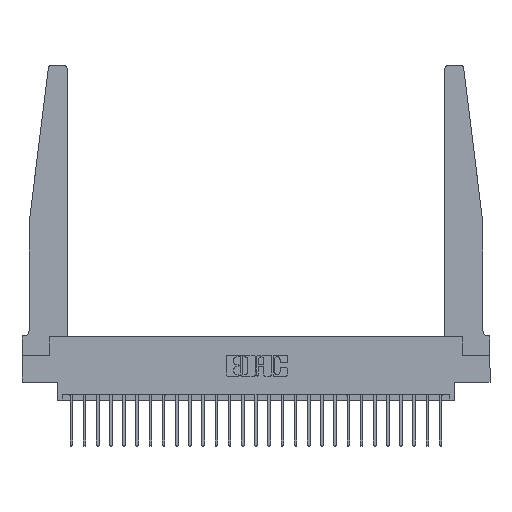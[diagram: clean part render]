
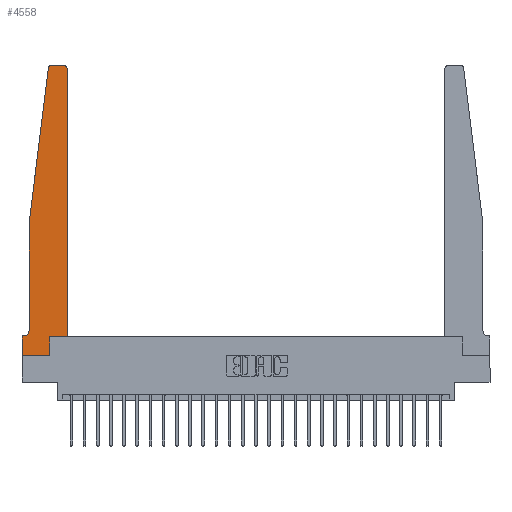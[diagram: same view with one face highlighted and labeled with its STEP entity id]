
A CAD part, top view. The second image highlights one B-rep face of the part: STEP entity #4558.
In plain terms, the highlighted planar face has unit normal (0, 0, 1).
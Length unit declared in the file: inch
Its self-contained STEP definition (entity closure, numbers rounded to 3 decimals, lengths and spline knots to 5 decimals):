
#84 = LINE ( 'NONE', #6139, #25958 ) ;
#349 = DIRECTION ( 'NONE',  ( 0., 0., -1. ) ) ;
#415 = CARTESIAN_POINT ( 'NONE',  ( 0.2605, 0.18, 0.37 ) ) ;
#795 = DIRECTION ( 'NONE',  ( 1., 0., 0. ) ) ;
#845 = VERTEX_POINT ( 'NONE', #19934 ) ;
#1404 = DIRECTION ( 'NONE',  ( 0., 0., 1. ) ) ;
#1995 = CIRCLE ( 'NONE', #16306, 0.03 ) ;
#2336 = CARTESIAN_POINT ( 'NONE',  ( 0.2605, 0.18, 0.37 ) ) ;
#2342 = CARTESIAN_POINT ( 'NONE',  ( 0.27653, 2.75, 0.37 ) ) ;
#2404 = ORIENTED_EDGE ( 'NONE', *, *, #10824, .T. ) ;
#3598 = VECTOR ( 'NONE', #15626, 39.37008 ) ;
#3661 = EDGE_CURVE ( 'NONE', #4424, #20110, #20264, .T. ) ;
#3955 = ORIENTED_EDGE ( 'NONE', *, *, #22838, .T. ) ;
#4188 = DIRECTION ( 'NONE',  ( 0., 1., 0. ) ) ;
#4293 = VECTOR ( 'NONE', #20482, 39.37008 ) ;
#4340 = EDGE_CURVE ( 'NONE', #5975, #11841, #15081, .T. ) ;
#4424 = VERTEX_POINT ( 'NONE', #20037 ) ;
#4433 = CARTESIAN_POINT ( 'NONE',  ( 0.395, 2.75, 0.37 ) ) ;
#4449 = CARTESIAN_POINT ( 'NONE',  ( 0.015, 0.1875, 0.37 ) ) ;
#4558 = ADVANCED_FACE ( 'NONE', ( #22544 ), #24651, .T. ) ;
#4831 = LINE ( 'NONE', #10779, #14802 ) ;
#5114 = VERTEX_POINT ( 'NONE', #4449 ) ;
#5836 = CARTESIAN_POINT ( 'NONE',  ( 0.065, 0.1875, 0.37 ) ) ;
#5975 = VERTEX_POINT ( 'NONE', #4433 ) ;
#6001 = DIRECTION ( 'NONE',  ( 0., -1., 0. ) ) ;
#6057 = CARTESIAN_POINT ( 'NONE',  ( 0.425, 2.72, 0.37 ) ) ;
#6135 = EDGE_CURVE ( 'NONE', #23276, #5975, #12417, .T. ) ;
#6139 = CARTESIAN_POINT ( 'NONE',  ( 0., 0., 0.37 ) ) ;
#6272 = DIRECTION ( 'NONE',  ( -1., 0., 0. ) ) ;
#6506 = CARTESIAN_POINT ( 'NONE',  ( 0.065, 1.25, 0.37 ) ) ;
#6802 = VERTEX_POINT ( 'NONE', #7889 ) ;
#6846 = DIRECTION ( 'NONE',  ( 0., 0., 1. ) ) ;
#7079 = DIRECTION ( 'NONE',  ( 0., 1., 0. ) ) ;
#7572 = DIRECTION ( 'NONE',  ( 1., 0., 0. ) ) ;
#7683 = LINE ( 'NONE', #15757, #3598 ) ;
#7856 = VERTEX_POINT ( 'NONE', #21136 ) ;
#7889 = CARTESIAN_POINT ( 'NONE',  ( 0.065, 1.25, 0.37 ) ) ;
#7890 = VECTOR ( 'NONE', #14556, 39.37008 ) ;
#9022 = VERTEX_POINT ( 'NONE', #21777 ) ;
#9404 = DIRECTION ( 'NONE',  ( -1., 0., 0. ) ) ;
#9525 = CIRCLE ( 'NONE', #19628, 0.05 ) ;
#9925 = ORIENTED_EDGE ( 'NONE', *, *, #20898, .T. ) ;
#10779 = CARTESIAN_POINT ( 'NONE',  ( 0.425, 0.18, 0.37 ) ) ;
#10824 = EDGE_CURVE ( 'NONE', #24375, #23276, #4831, .T. ) ;
#11055 = ORIENTED_EDGE ( 'NONE', *, *, #20810, .T. ) ;
#11338 = EDGE_CURVE ( 'NONE', #22339, #6802, #18080, .T. ) ;
#11629 = ORIENTED_EDGE ( 'NONE', *, *, #6135, .T. ) ;
#11781 = LINE ( 'NONE', #5836, #16328 ) ;
#11841 = VERTEX_POINT ( 'NONE', #2342 ) ;
#12039 = LINE ( 'NONE', #16641, #7890 ) ;
#12293 = VECTOR ( 'NONE', #4188, 39.37008 ) ;
#12417 = CIRCLE ( 'NONE', #15789, 0.03 ) ;
#13108 = ORIENTED_EDGE ( 'NONE', *, *, #22732, .T. ) ;
#13673 = EDGE_CURVE ( 'NONE', #6802, #7856, #14440, .T. ) ;
#13743 = CARTESIAN_POINT ( 'NONE',  ( 0.065, 1.25, 0.37 ) ) ;
#13976 = VECTOR ( 'NONE', #19778, 39.37008 ) ;
#14281 = ORIENTED_EDGE ( 'NONE', *, *, #11338, .T. ) ;
#14440 = LINE ( 'NONE', #6506, #4293 ) ;
#14556 = DIRECTION ( 'NONE',  ( 1., 0., 0. ) ) ;
#14802 = VECTOR ( 'NONE', #7079, 39.37008 ) ;
#15081 = LINE ( 'NONE', #25474, #25430 ) ;
#15377 = CARTESIAN_POINT ( 'NONE',  ( 0.395, 2.72, 0.37 ) ) ;
#15550 = CARTESIAN_POINT ( 'NONE',  ( 0.27653, 2.72, 0.37 ) ) ;
#15626 = DIRECTION ( 'NONE',  ( 1., 0., 0. ) ) ;
#15757 = CARTESIAN_POINT ( 'NONE',  ( 0.425, 0.18, 0.37 ) ) ;
#15789 = AXIS2_PLACEMENT_3D ( 'NONE', #15377, #1404, #7572 ) ;
#15913 = ORIENTED_EDGE ( 'NONE', *, *, #3661, .T. ) ;
#16302 = CARTESIAN_POINT ( 'NONE',  ( 0.015, 0.2375, 0.37 ) ) ;
#16306 = AXIS2_PLACEMENT_3D ( 'NONE', #15550, #19610, #23430 ) ;
#16328 = VECTOR ( 'NONE', #9404, 39.37008 ) ;
#16641 = CARTESIAN_POINT ( 'NONE',  ( 0., 0., 0.37 ) ) ;
#17316 = ORIENTED_EDGE ( 'NONE', *, *, #22232, .T. ) ;
#18080 = LINE ( 'NONE', #13743, #13976 ) ;
#18154 = EDGE_CURVE ( 'NONE', #20110, #24375, #7683, .T. ) ;
#19610 = DIRECTION ( 'NONE',  ( 0., 0., 1. ) ) ;
#19628 = AXIS2_PLACEMENT_3D ( 'NONE', #16302, #349, #6272 ) ;
#19778 = DIRECTION ( 'NONE',  ( -0.122, -0.992, 0. ) ) ;
#19934 = CARTESIAN_POINT ( 'NONE',  ( 0., 0.1875, 0.37 ) ) ;
#20037 = CARTESIAN_POINT ( 'NONE',  ( 0.2605, 0., 0.37 ) ) ;
#20110 = VERTEX_POINT ( 'NONE', #415 ) ;
#20264 = LINE ( 'NONE', #2336, #12293 ) ;
#20482 = DIRECTION ( 'NONE',  ( 0., -1., 0. ) ) ;
#20810 = EDGE_CURVE ( 'NONE', #7856, #5114, #9525, .T. ) ;
#20898 = EDGE_CURVE ( 'NONE', #845, #9022, #84, .T. ) ;
#21136 = CARTESIAN_POINT ( 'NONE',  ( 0.065, 0.2375, 0.37 ) ) ;
#21592 = CARTESIAN_POINT ( 'NONE',  ( 0.24675, 2.72367, 0.37 ) ) ;
#21777 = CARTESIAN_POINT ( 'NONE',  ( 0., 0., 0.37 ) ) ;
#22056 = ORIENTED_EDGE ( 'NONE', *, *, #13673, .T. ) ;
#22232 = EDGE_CURVE ( 'NONE', #11841, #22339, #1995, .T. ) ;
#22339 = VERTEX_POINT ( 'NONE', #21592 ) ;
#22544 = FACE_OUTER_BOUND ( 'NONE', #23392, .T. ) ;
#22732 = EDGE_CURVE ( 'NONE', #5114, #845, #11781, .T. ) ;
#22797 = CARTESIAN_POINT ( 'NONE',  ( 0., 0.1875, 0.37 ) ) ;
#22838 = EDGE_CURVE ( 'NONE', #9022, #4424, #12039, .T. ) ;
#22987 = CARTESIAN_POINT ( 'NONE',  ( 0.425, 0.18, 0.37 ) ) ;
#23082 = DIRECTION ( 'NONE',  ( -1., 0., 0. ) ) ;
#23276 = VERTEX_POINT ( 'NONE', #6057 ) ;
#23392 = EDGE_LOOP ( 'NONE', ( #25286, #17316, #14281, #22056, #11055, #13108, #9925, #3955, #15913, #25673, #2404, #11629 ) ) ;
#23430 = DIRECTION ( 'NONE',  ( 1., 0., 0. ) ) ;
#24375 = VERTEX_POINT ( 'NONE', #22987 ) ;
#24593 = AXIS2_PLACEMENT_3D ( 'NONE', #22797, #6846, #795 ) ;
#24651 = PLANE ( 'NONE',  #24593 ) ;
#25286 = ORIENTED_EDGE ( 'NONE', *, *, #4340, .T. ) ;
#25430 = VECTOR ( 'NONE', #23082, 39.37008 ) ;
#25474 = CARTESIAN_POINT ( 'NONE',  ( 0.25, 2.75, 0.37 ) ) ;
#25673 = ORIENTED_EDGE ( 'NONE', *, *, #18154, .T. ) ;
#25958 = VECTOR ( 'NONE', #6001, 39.37008 ) ;
